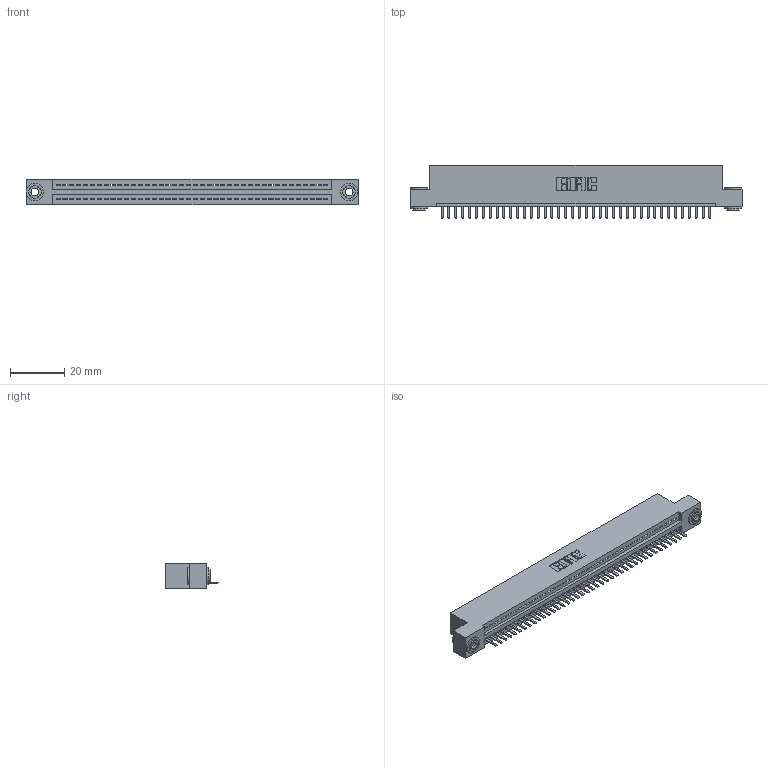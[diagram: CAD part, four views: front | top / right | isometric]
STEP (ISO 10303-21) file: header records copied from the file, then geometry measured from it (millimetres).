
FILE_DESCRIPTION (( 'STEP AP203' ), '1' );
FILE_NAME ('345-040-520-103.STEP', '2018-09-05T00:50:35', ( '' ), ( '' ), 'SwSTEP 2.0', 'SolidWorks 2016', '' );
FILE_SCHEMA (( 'CONFIG_CONTROL_DESIGN' ));
Length unit declared in the file: inch
Products named in the file (4): 345-040-520-103; 345 Part_Flush Mounting Lugs - 0.156 Dia-TH; 345-292-001_345-293-120; 345-250-002_345-250-002-102
Assembly tree (43 placements, depth 2):
  345-040-520-103
    345 Part_Flush Mounting Lugs - 0.156 Dia-TH
    345-292-001_345-293-120  x40
    345-250-002_345-250-002-102  x2
Bounding box: 122.81 x 19.68 x 9.4 mm (x, y, z)
Volume: 11552.5 mm3; surface area: 15163.1 mm2
Topology: 43 solids, 43 shells, 2644 faces, 7777 edges, 5074 vertices
Faces by surface type: plane 1770, cylinder 866, cone 8
Entity records: 31138 total; most frequent: CARTESIAN_POINT 5383, ORIENTED_EDGE 5338, DIRECTION 4723, EDGE_CURVE 2669, LINE 2349, VECTOR 2349, VERTEX_POINT 1774, AXIS2_PLACEMENT_3D 1187
